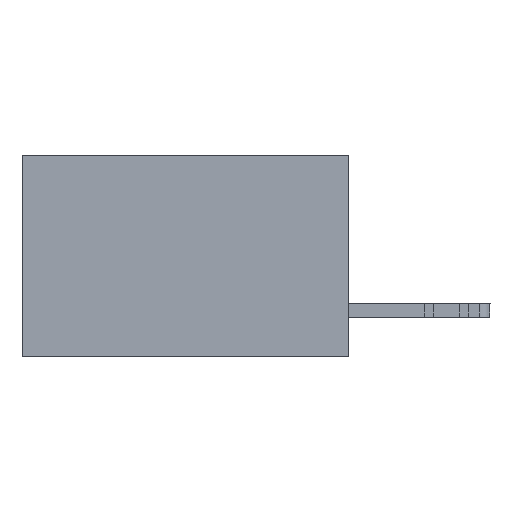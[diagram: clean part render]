
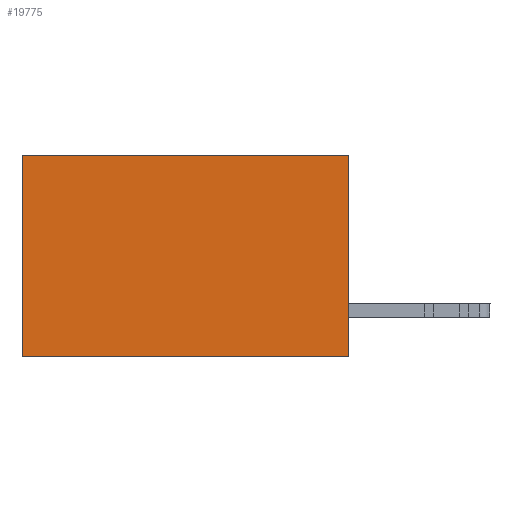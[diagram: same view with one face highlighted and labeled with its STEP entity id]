
A CAD part, left-side view. The second image highlights one B-rep face of the part: STEP entity #19775.
In plain terms, the highlighted planar face has unit normal (-1, 0, 0).
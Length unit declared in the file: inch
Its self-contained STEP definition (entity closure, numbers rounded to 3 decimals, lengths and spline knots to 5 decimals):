
#144 = VECTOR ( 'NONE', #18094, 39.37008 ) ;
#343 = EDGE_CURVE ( 'NONE', #15690, #10870, #15005, .T. ) ;
#2853 = VECTOR ( 'NONE', #9853, 39.37008 ) ;
#5559 = ORIENTED_EDGE ( 'NONE', *, *, #343, .T. ) ;
#6769 = CARTESIAN_POINT ( 'NONE',  ( 0.298, 0., 0. ) ) ;
#8963 = EDGE_CURVE ( 'NONE', #15690, #12819, #25388, .T. ) ;
#9853 = DIRECTION ( 'NONE',  ( 0., 1., 0. ) ) ;
#10040 = CARTESIAN_POINT ( 'NONE',  ( 0.298, 0.6, 0. ) ) ;
#10870 = VERTEX_POINT ( 'NONE', #22095 ) ;
#11438 = CARTESIAN_POINT ( 'NONE',  ( 0.298, 0., 0. ) ) ;
#11468 = CARTESIAN_POINT ( 'NONE',  ( 0.298, 0.6, -0.37 ) ) ;
#12793 = CARTESIAN_POINT ( 'NONE',  ( 0.298, 0., 0. ) ) ;
#12819 = VERTEX_POINT ( 'NONE', #28949 ) ;
#13411 = ORIENTED_EDGE ( 'NONE', *, *, #29201, .F. ) ;
#13542 = DIRECTION ( 'NONE',  ( 0., 0., -1. ) ) ;
#15005 = LINE ( 'NONE', #12793, #144 ) ;
#15507 = VECTOR ( 'NONE', #19114, 39.37008 ) ;
#15690 = VERTEX_POINT ( 'NONE', #30819 ) ;
#18094 = DIRECTION ( 'NONE',  ( 0., 1., 0. ) ) ;
#18108 = ORIENTED_EDGE ( 'NONE', *, *, #8963, .F. ) ;
#18212 = VERTEX_POINT ( 'NONE', #11468 ) ;
#18980 = EDGE_CURVE ( 'NONE', #10870, #18212, #26146, .T. ) ;
#19114 = DIRECTION ( 'NONE',  ( 0., 0., -1. ) ) ;
#19271 = ORIENTED_EDGE ( 'NONE', *, *, #18980, .T. ) ;
#19716 = DIRECTION ( 'NONE',  ( 0., 0., -1. ) ) ;
#19775 = ADVANCED_FACE ( 'NONE', ( #23433 ), #25674, .F. ) ;
#22095 = CARTESIAN_POINT ( 'NONE',  ( 0.298, 0.6, 0. ) ) ;
#22731 = VECTOR ( 'NONE', #19716, 39.37008 ) ;
#23229 = DIRECTION ( 'NONE',  ( 1., 0., 0. ) ) ;
#23433 = FACE_OUTER_BOUND ( 'NONE', #29999, .T. ) ;
#24559 = LINE ( 'NONE', #29074, #2853 ) ;
#25388 = LINE ( 'NONE', #6769, #15507 ) ;
#25674 = PLANE ( 'NONE',  #28946 ) ;
#26146 = LINE ( 'NONE', #10040, #22731 ) ;
#28946 = AXIS2_PLACEMENT_3D ( 'NONE', #11438, #23229, #13542 ) ;
#28949 = CARTESIAN_POINT ( 'NONE',  ( 0.298, 0., -0.37 ) ) ;
#29074 = CARTESIAN_POINT ( 'NONE',  ( 0.298, 0., -0.37 ) ) ;
#29201 = EDGE_CURVE ( 'NONE', #12819, #18212, #24559, .T. ) ;
#29999 = EDGE_LOOP ( 'NONE', ( #19271, #13411, #18108, #5559 ) ) ;
#30819 = CARTESIAN_POINT ( 'NONE',  ( 0.298, 0., 0. ) ) ;
